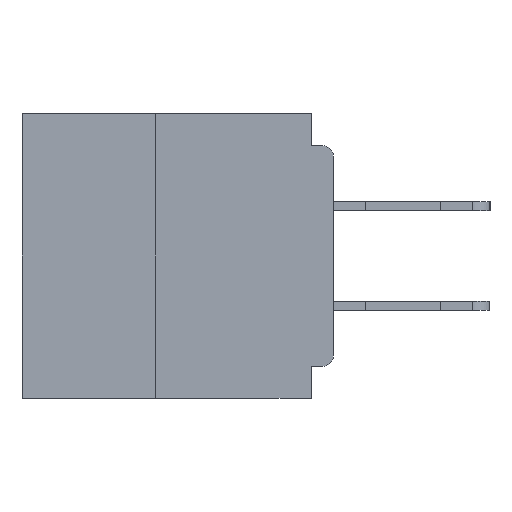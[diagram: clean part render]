
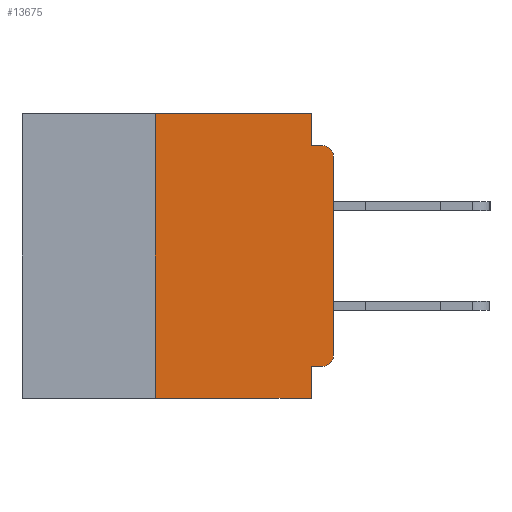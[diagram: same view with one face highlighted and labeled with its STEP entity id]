
A CAD part, left-side view. The second image highlights one B-rep face of the part: STEP entity #13675.
In plain terms, the highlighted planar face has unit normal (-1, 0, 0).
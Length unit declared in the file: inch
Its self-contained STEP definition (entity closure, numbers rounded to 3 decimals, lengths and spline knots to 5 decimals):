
#333 = VERTEX_POINT ( 'NONE', #4917 ) ;
#776 = VECTOR ( 'NONE', #12939, 39.37008 ) ;
#864 = EDGE_CURVE ( 'NONE', #15130, #11704, #22920, .T. ) ;
#2947 = DIRECTION ( 'NONE',  ( 0., 0., -1. ) ) ;
#4334 = EDGE_CURVE ( 'NONE', #333, #4369, #23700, .T. ) ;
#4369 = VERTEX_POINT ( 'NONE', #44150 ) ;
#4917 = CARTESIAN_POINT ( 'NONE',  ( 0., 0.25, -0.4 ) ) ;
#5094 = VECTOR ( 'NONE', #16802, 39.37008 ) ;
#5414 = EDGE_CURVE ( 'NONE', #23885, #8152, #25244, .T. ) ;
#5511 = EDGE_CURVE ( 'NONE', #30896, #23750, #10190, .T. ) ;
#6348 = CARTESIAN_POINT ( 'NONE',  ( 0., 0.031, -0.355 ) ) ;
#6702 = EDGE_CURVE ( 'NONE', #11704, #26062, #22133, .T. ) ;
#6907 = VECTOR ( 'NONE', #18488, 39.37008 ) ;
#8060 = CARTESIAN_POINT ( 'NONE',  ( 0., 0.015, -0.045 ) ) ;
#8111 = AXIS2_PLACEMENT_3D ( 'NONE', #15461, #15935, #15574 ) ;
#8152 = VERTEX_POINT ( 'NONE', #34231 ) ;
#8323 = VECTOR ( 'NONE', #37124, 39.37008 ) ;
#9342 = CARTESIAN_POINT ( 'NONE',  ( 0., 0.031, 0. ) ) ;
#10190 = LINE ( 'NONE', #31270, #37364 ) ;
#11032 = EDGE_CURVE ( 'NONE', #23750, #4369, #17799, .T. ) ;
#11405 = CARTESIAN_POINT ( 'NONE',  ( 0., 0., -0.34 ) ) ;
#11704 = VERTEX_POINT ( 'NONE', #19614 ) ;
#12000 = AXIS2_PLACEMENT_3D ( 'NONE', #37876, #16681, #41386 ) ;
#12939 = DIRECTION ( 'NONE',  ( 0., 0., -1. ) ) ;
#13675 = ADVANCED_FACE ( 'NONE', ( #25976 ), #20717, .F. ) ;
#13682 = EDGE_CURVE ( 'NONE', #14523, #26062, #35340, .T. ) ;
#14350 = EDGE_LOOP ( 'NONE', ( #22457, #33777, #28782, #39427, #28259, #39794, #39610, #39024, #39656, #31323 ) ) ;
#14523 = VERTEX_POINT ( 'NONE', #22333 ) ;
#15130 = VERTEX_POINT ( 'NONE', #11405 ) ;
#15461 = CARTESIAN_POINT ( 'NONE',  ( 0., 0.015, -0.06 ) ) ;
#15574 = DIRECTION ( 'NONE',  ( 0., 0., -1. ) ) ;
#15935 = DIRECTION ( 'NONE',  ( -1., 0., 0. ) ) ;
#16681 = DIRECTION ( 'NONE',  ( -1., 0., 0. ) ) ;
#16802 = DIRECTION ( 'NONE',  ( 0., 0., 1. ) ) ;
#17119 = DIRECTION ( 'NONE',  ( 0., -1., 0. ) ) ;
#17799 = LINE ( 'NONE', #22925, #8323 ) ;
#18488 = DIRECTION ( 'NONE',  ( 0., 0., 1. ) ) ;
#19345 = CARTESIAN_POINT ( 'NONE',  ( 0., 0.015, -0.355 ) ) ;
#19614 = CARTESIAN_POINT ( 'NONE',  ( 0., 0., -0.06 ) ) ;
#20717 = PLANE ( 'NONE',  #23845 ) ;
#20871 = EDGE_CURVE ( 'NONE', #8152, #14523, #28067, .T. ) ;
#21302 = CARTESIAN_POINT ( 'NONE',  ( 0., 0.25, 0. ) ) ;
#22133 = CIRCLE ( 'NONE', #8111, 0.015 ) ;
#22333 = CARTESIAN_POINT ( 'NONE',  ( 0., 0.031, -0.045 ) ) ;
#22457 = ORIENTED_EDGE ( 'NONE', *, *, #864, .T. ) ;
#22920 = LINE ( 'NONE', #24743, #5094 ) ;
#22925 = CARTESIAN_POINT ( 'NONE',  ( 0., 0.031, -0.4 ) ) ;
#23700 = LINE ( 'NONE', #45707, #42406 ) ;
#23750 = VERTEX_POINT ( 'NONE', #6348 ) ;
#23845 = AXIS2_PLACEMENT_3D ( 'NONE', #41823, #24275, #2947 ) ;
#23885 = VERTEX_POINT ( 'NONE', #21302 ) ;
#24151 = VECTOR ( 'NONE', #35013, 39.37008 ) ;
#24275 = DIRECTION ( 'NONE',  ( 1., 0., 0. ) ) ;
#24743 = CARTESIAN_POINT ( 'NONE',  ( 0., 0., 0. ) ) ;
#25244 = LINE ( 'NONE', #35257, #24151 ) ;
#25685 = EDGE_CURVE ( 'NONE', #30896, #15130, #25695, .T. ) ;
#25695 = CIRCLE ( 'NONE', #12000, 0.015 ) ;
#25976 = FACE_OUTER_BOUND ( 'NONE', #14350, .T. ) ;
#26062 = VERTEX_POINT ( 'NONE', #8060 ) ;
#27856 = CARTESIAN_POINT ( 'NONE',  ( 0., 0., -0.045 ) ) ;
#28067 = LINE ( 'NONE', #9342, #776 ) ;
#28259 = ORIENTED_EDGE ( 'NONE', *, *, #5414, .F. ) ;
#28782 = ORIENTED_EDGE ( 'NONE', *, *, #13682, .F. ) ;
#30166 = EDGE_CURVE ( 'NONE', #333, #23885, #42377, .T. ) ;
#30896 = VERTEX_POINT ( 'NONE', #19345 ) ;
#31270 = CARTESIAN_POINT ( 'NONE',  ( 0., 0., -0.355 ) ) ;
#31323 = ORIENTED_EDGE ( 'NONE', *, *, #25685, .T. ) ;
#31472 = DIRECTION ( 'NONE',  ( 0., 1., 0. ) ) ;
#33777 = ORIENTED_EDGE ( 'NONE', *, *, #6702, .T. ) ;
#34231 = CARTESIAN_POINT ( 'NONE',  ( 0., 0.031, 0. ) ) ;
#35013 = DIRECTION ( 'NONE',  ( 0., -1., 0. ) ) ;
#35257 = CARTESIAN_POINT ( 'NONE',  ( 0., 0.437, 0. ) ) ;
#35340 = LINE ( 'NONE', #27856, #43562 ) ;
#37124 = DIRECTION ( 'NONE',  ( 0., 0., -1. ) ) ;
#37364 = VECTOR ( 'NONE', #31472, 39.37008 ) ;
#37876 = CARTESIAN_POINT ( 'NONE',  ( 0., 0.015, -0.34 ) ) ;
#39024 = ORIENTED_EDGE ( 'NONE', *, *, #11032, .F. ) ;
#39427 = ORIENTED_EDGE ( 'NONE', *, *, #20871, .F. ) ;
#39610 = ORIENTED_EDGE ( 'NONE', *, *, #4334, .T. ) ;
#39632 = CARTESIAN_POINT ( 'NONE',  ( 0., 0.25, -0.4 ) ) ;
#39656 = ORIENTED_EDGE ( 'NONE', *, *, #5511, .F. ) ;
#39794 = ORIENTED_EDGE ( 'NONE', *, *, #30166, .F. ) ;
#41386 = DIRECTION ( 'NONE',  ( 0., 0., -1. ) ) ;
#41823 = CARTESIAN_POINT ( 'NONE',  ( 0., 0.437, 0. ) ) ;
#42377 = LINE ( 'NONE', #39632, #6907 ) ;
#42406 = VECTOR ( 'NONE', #45606, 39.37008 ) ;
#43562 = VECTOR ( 'NONE', #17119, 39.37008 ) ;
#44150 = CARTESIAN_POINT ( 'NONE',  ( 0., 0.031, -0.4 ) ) ;
#45606 = DIRECTION ( 'NONE',  ( 0., -1., 0. ) ) ;
#45707 = CARTESIAN_POINT ( 'NONE',  ( 0., 0.437, -0.4 ) ) ;
